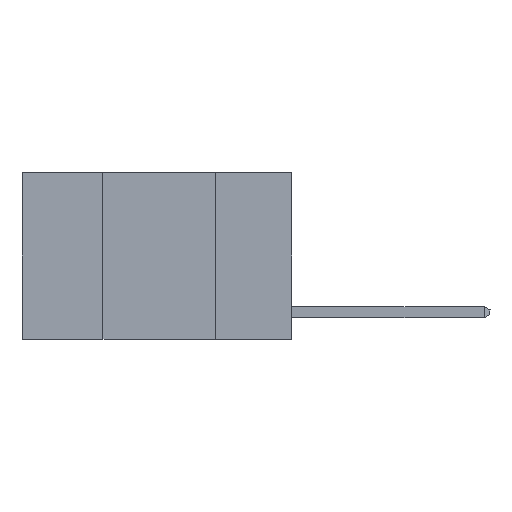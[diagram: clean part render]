
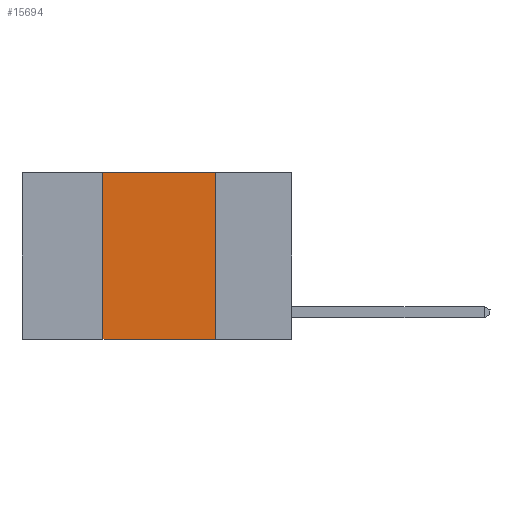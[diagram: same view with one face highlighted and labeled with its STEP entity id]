
A CAD part, left-side view. The second image highlights one B-rep face of the part: STEP entity #15694.
In plain terms, the highlighted planar face has unit normal (-1, 0, 0).
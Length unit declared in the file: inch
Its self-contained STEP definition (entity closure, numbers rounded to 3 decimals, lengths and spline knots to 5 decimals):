
#654 = CARTESIAN_POINT ( 'NONE',  ( 0., 0.42, 0. ) ) ;
#727 = EDGE_CURVE ( 'NONE', #11465, #17570, #21946, .T. ) ;
#1980 = EDGE_CURVE ( 'NONE', #9869, #19405, #10107, .T. ) ;
#2312 = CARTESIAN_POINT ( 'NONE',  ( 0., 0.17, 0. ) ) ;
#2793 = VECTOR ( 'NONE', #20205, 39.37008 ) ;
#3416 = CARTESIAN_POINT ( 'NONE',  ( 0., 0.17, -0.37 ) ) ;
#3966 = CARTESIAN_POINT ( 'NONE',  ( 0., 0.42, 0. ) ) ;
#5238 = VECTOR ( 'NONE', #20304, 39.37008 ) ;
#7812 = LINE ( 'NONE', #23829, #2793 ) ;
#8708 = VECTOR ( 'NONE', #21341, 39.37008 ) ;
#9005 = PLANE ( 'NONE',  #23649 ) ;
#9436 = ORIENTED_EDGE ( 'NONE', *, *, #727, .F. ) ;
#9869 = VERTEX_POINT ( 'NONE', #12130 ) ;
#10107 = LINE ( 'NONE', #23106, #17214 ) ;
#11383 = EDGE_CURVE ( 'NONE', #17570, #19405, #7812, .T. ) ;
#11465 = VERTEX_POINT ( 'NONE', #3966 ) ;
#12130 = CARTESIAN_POINT ( 'NONE',  ( 0., 0.42, -0.37 ) ) ;
#12772 = ORIENTED_EDGE ( 'NONE', *, *, #1980, .T. ) ;
#13671 = LINE ( 'NONE', #654, #8708 ) ;
#15694 = ADVANCED_FACE ( 'NONE', ( #22839 ), #9005, .F. ) ;
#16461 = EDGE_LOOP ( 'NONE', ( #17952, #9436, #18080, #12772 ) ) ;
#17214 = VECTOR ( 'NONE', #23434, 39.37008 ) ;
#17570 = VERTEX_POINT ( 'NONE', #2312 ) ;
#17952 = ORIENTED_EDGE ( 'NONE', *, *, #11383, .F. ) ;
#18080 = ORIENTED_EDGE ( 'NONE', *, *, #19135, .F. ) ;
#18535 = DIRECTION ( 'NONE',  ( 1., 0., 0. ) ) ;
#19135 = EDGE_CURVE ( 'NONE', #9869, #11465, #13671, .T. ) ;
#19405 = VERTEX_POINT ( 'NONE', #3416 ) ;
#20205 = DIRECTION ( 'NONE',  ( 0., 0., -1. ) ) ;
#20304 = DIRECTION ( 'NONE',  ( 0., -1., 0. ) ) ;
#20393 = DIRECTION ( 'NONE',  ( 0., 0., -1. ) ) ;
#20471 = CARTESIAN_POINT ( 'NONE',  ( 0., 0.6, 0. ) ) ;
#21341 = DIRECTION ( 'NONE',  ( 0., 0., 1. ) ) ;
#21946 = LINE ( 'NONE', #22097, #5238 ) ;
#22097 = CARTESIAN_POINT ( 'NONE',  ( 0., 0.6, 0. ) ) ;
#22839 = FACE_OUTER_BOUND ( 'NONE', #16461, .T. ) ;
#23106 = CARTESIAN_POINT ( 'NONE',  ( 0., 0.6, -0.37 ) ) ;
#23434 = DIRECTION ( 'NONE',  ( 0., -1., 0. ) ) ;
#23649 = AXIS2_PLACEMENT_3D ( 'NONE', #20471, #18535, #20393 ) ;
#23829 = CARTESIAN_POINT ( 'NONE',  ( 0., 0.17, 0. ) ) ;
